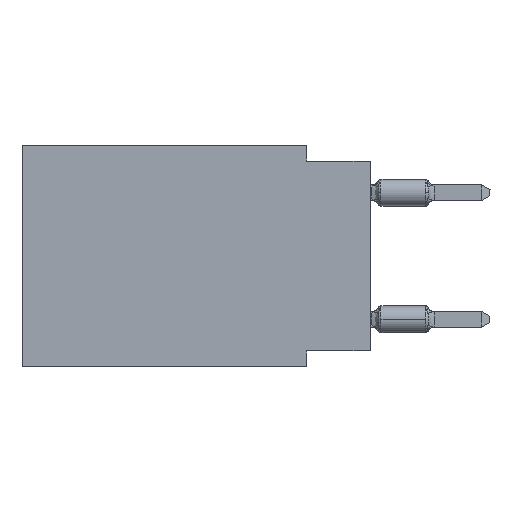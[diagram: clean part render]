
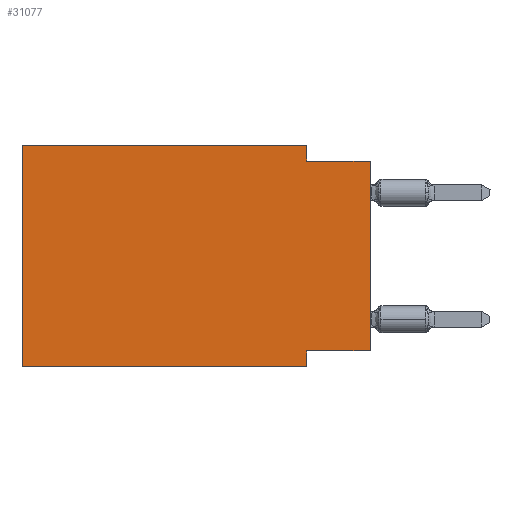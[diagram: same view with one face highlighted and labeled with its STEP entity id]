
A CAD part, left-side view. The second image highlights one B-rep face of the part: STEP entity #31077.
In plain terms, the highlighted planar face has unit normal (-1, 0, 0).
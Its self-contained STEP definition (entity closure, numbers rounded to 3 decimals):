
#195 = EDGE_CURVE ( 'NONE', #36139, #29900, #34089, .T. ) ;
#1619 = EDGE_CURVE ( 'NONE', #3235, #29900, #30720, .T. ) ;
#1803 = DIRECTION ( 'NONE',  ( 0., -1., 0. ) ) ;
#2967 = VECTOR ( 'NONE', #18657, 1000. ) ;
#3235 = VERTEX_POINT ( 'NONE', #15899 ) ;
#3355 = VECTOR ( 'NONE', #1803, 1000. ) ;
#3871 = EDGE_LOOP ( 'NONE', ( #23585, #26561, #7430, #33840, #18082, #21958, #38260, #40732 ) ) ;
#3921 = CARTESIAN_POINT ( 'NONE',  ( 0., 0., -8.255 ) ) ;
#4052 = CARTESIAN_POINT ( 'NONE',  ( 0., 2.54, 0. ) ) ;
#4117 = VECTOR ( 'NONE', #25382, 1000. ) ;
#4129 = PLANE ( 'NONE',  #18986 ) ;
#4265 = CARTESIAN_POINT ( 'NONE',  ( 0., 2.54, -0.635 ) ) ;
#4961 = CARTESIAN_POINT ( 'NONE',  ( 0., 2.54, -8.89 ) ) ;
#5437 = VERTEX_POINT ( 'NONE', #4265 ) ;
#7430 = ORIENTED_EDGE ( 'NONE', *, *, #12421, .F. ) ;
#7936 = CARTESIAN_POINT ( 'NONE',  ( 0., 2.54, -8.89 ) ) ;
#9891 = VECTOR ( 'NONE', #30278, 1000. ) ;
#10023 = LINE ( 'NONE', #22996, #18998 ) ;
#10061 = CARTESIAN_POINT ( 'NONE',  ( 0., 13.97, 0. ) ) ;
#10931 = LINE ( 'NONE', #40281, #9891 ) ;
#11763 = CARTESIAN_POINT ( 'NONE',  ( 0., 0., -8.255 ) ) ;
#12421 = EDGE_CURVE ( 'NONE', #21708, #5437, #39555, .T. ) ;
#13143 = VECTOR ( 'NONE', #26026, 1000. ) ;
#13463 = VECTOR ( 'NONE', #40189, 1000. ) ;
#13691 = DIRECTION ( 'NONE',  ( 1., 0., 0. ) ) ;
#14045 = CARTESIAN_POINT ( 'NONE',  ( 0., 0., -0.635 ) ) ;
#14176 = CARTESIAN_POINT ( 'NONE',  ( 0., 2.54, 0. ) ) ;
#15899 = CARTESIAN_POINT ( 'NONE',  ( 0., 13.97, -8.89 ) ) ;
#17923 = DIRECTION ( 'NONE',  ( 0., 0., -1. ) ) ;
#18082 = ORIENTED_EDGE ( 'NONE', *, *, #25731, .F. ) ;
#18196 = VECTOR ( 'NONE', #17923, 1000. ) ;
#18657 = DIRECTION ( 'NONE',  ( 0., 0., 1. ) ) ;
#18986 = AXIS2_PLACEMENT_3D ( 'NONE', #33670, #13691, #39632 ) ;
#18998 = VECTOR ( 'NONE', #32991, 1000. ) ;
#19648 = LINE ( 'NONE', #10061, #4117 ) ;
#20490 = CARTESIAN_POINT ( 'NONE',  ( 0., 13.97, 0. ) ) ;
#20919 = EDGE_CURVE ( 'NONE', #27861, #25081, #10931, .T. ) ;
#21130 = FACE_OUTER_BOUND ( 'NONE', #3871, .T. ) ;
#21708 = VERTEX_POINT ( 'NONE', #14176 ) ;
#21958 = ORIENTED_EDGE ( 'NONE', *, *, #1619, .T. ) ;
#22996 = CARTESIAN_POINT ( 'NONE',  ( 0., 0., -0.635 ) ) ;
#23585 = ORIENTED_EDGE ( 'NONE', *, *, #20919, .T. ) ;
#25081 = VERTEX_POINT ( 'NONE', #14045 ) ;
#25382 = DIRECTION ( 'NONE',  ( 0., -1., 0. ) ) ;
#25731 = EDGE_CURVE ( 'NONE', #3235, #34819, #38838, .T. ) ;
#26026 = DIRECTION ( 'NONE',  ( 0., 1., 0. ) ) ;
#26365 = EDGE_CURVE ( 'NONE', #27861, #36139, #35605, .T. ) ;
#26561 = ORIENTED_EDGE ( 'NONE', *, *, #37162, .F. ) ;
#27861 = VERTEX_POINT ( 'NONE', #11763 ) ;
#28432 = EDGE_CURVE ( 'NONE', #34819, #21708, #19648, .T. ) ;
#28833 = CARTESIAN_POINT ( 'NONE',  ( 0., 2.54, -8.255 ) ) ;
#29900 = VERTEX_POINT ( 'NONE', #7936 ) ;
#30278 = DIRECTION ( 'NONE',  ( 0., 0., 1. ) ) ;
#30720 = LINE ( 'NONE', #40489, #3355 ) ;
#31077 = ADVANCED_FACE ( 'NONE', ( #21130 ), #4129, .F. ) ;
#32991 = DIRECTION ( 'NONE',  ( 0., -1., 0. ) ) ;
#33670 = CARTESIAN_POINT ( 'NONE',  ( 0., 13.97, 0. ) ) ;
#33840 = ORIENTED_EDGE ( 'NONE', *, *, #28432, .F. ) ;
#34089 = LINE ( 'NONE', #4961, #18196 ) ;
#34819 = VERTEX_POINT ( 'NONE', #20490 ) ;
#35605 = LINE ( 'NONE', #3921, #13143 ) ;
#36139 = VERTEX_POINT ( 'NONE', #28833 ) ;
#37162 = EDGE_CURVE ( 'NONE', #5437, #25081, #10023, .T. ) ;
#38260 = ORIENTED_EDGE ( 'NONE', *, *, #195, .F. ) ;
#38406 = CARTESIAN_POINT ( 'NONE',  ( 0., 13.97, 0. ) ) ;
#38838 = LINE ( 'NONE', #38406, #2967 ) ;
#39555 = LINE ( 'NONE', #4052, #13463 ) ;
#39632 = DIRECTION ( 'NONE',  ( 0., 0., -1. ) ) ;
#40189 = DIRECTION ( 'NONE',  ( 0., 0., -1. ) ) ;
#40281 = CARTESIAN_POINT ( 'NONE',  ( 0., 0., 0. ) ) ;
#40489 = CARTESIAN_POINT ( 'NONE',  ( 0., 13.97, -8.89 ) ) ;
#40732 = ORIENTED_EDGE ( 'NONE', *, *, #26365, .F. ) ;
